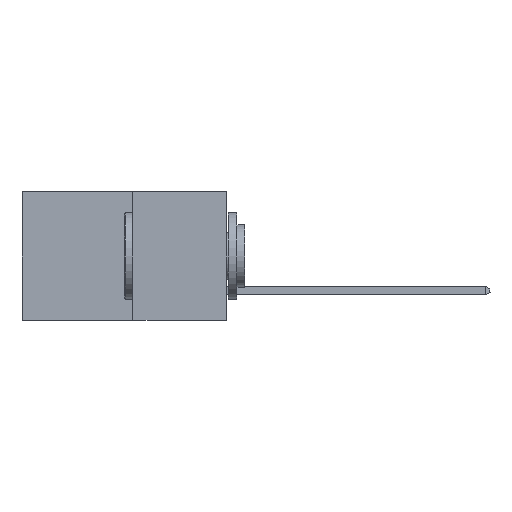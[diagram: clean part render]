
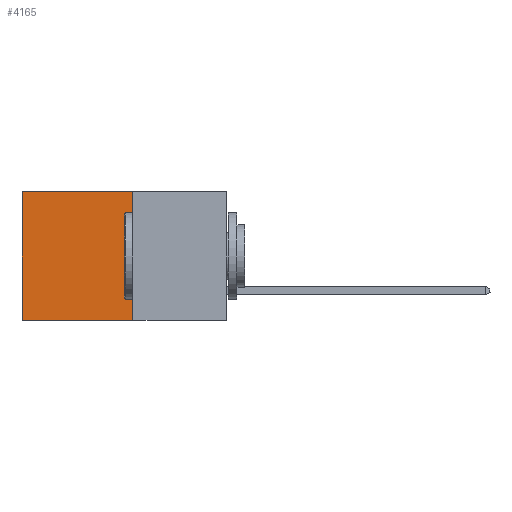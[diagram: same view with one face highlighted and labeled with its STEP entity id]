
A CAD part, left-side view. The second image highlights one B-rep face of the part: STEP entity #4165.
In plain terms, the highlighted planar face has unit normal (-1, 0, 0).
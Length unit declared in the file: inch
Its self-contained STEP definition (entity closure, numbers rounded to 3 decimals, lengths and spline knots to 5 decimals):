
#2106 = ORIENTED_EDGE ( 'NONE', *, *, #10642, .T. ) ;
#2126 = VERTEX_POINT ( 'NONE', #22899 ) ;
#2485 = CARTESIAN_POINT ( 'NONE',  ( 0.277, 0.27, -0.37 ) ) ;
#2646 = DIRECTION ( 'NONE',  ( 0., 0., -1. ) ) ;
#3081 = VECTOR ( 'NONE', #4886, 39.37008 ) ;
#3517 = CARTESIAN_POINT ( 'NONE',  ( 0.277, 0.27, 0. ) ) ;
#4165 = ADVANCED_FACE ( 'NONE', ( #8688 ), #10980, .F. ) ;
#4886 = DIRECTION ( 'NONE',  ( 0., 0., -1. ) ) ;
#5618 = LINE ( 'NONE', #25463, #28935 ) ;
#5661 = ORIENTED_EDGE ( 'NONE', *, *, #24404, .F. ) ;
#6043 = CARTESIAN_POINT ( 'NONE',  ( 0.277, 0.27, -0.37 ) ) ;
#6170 = CARTESIAN_POINT ( 'NONE',  ( 0.277, 0.27, -0.37 ) ) ;
#6928 = CARTESIAN_POINT ( 'NONE',  ( 0.277, 0.59, 0. ) ) ;
#7022 = ORIENTED_EDGE ( 'NONE', *, *, #10318, .T. ) ;
#8307 = LINE ( 'NONE', #17026, #26738 ) ;
#8645 = DIRECTION ( 'NONE',  ( 0., 1., 0. ) ) ;
#8688 = FACE_OUTER_BOUND ( 'NONE', #18865, .T. ) ;
#9369 = VERTEX_POINT ( 'NONE', #6170 ) ;
#10318 = EDGE_CURVE ( 'NONE', #23981, #2126, #8307, .T. ) ;
#10642 = EDGE_CURVE ( 'NONE', #29836, #23981, #5618, .T. ) ;
#10799 = DIRECTION ( 'NONE',  ( 0., 0., -1. ) ) ;
#10828 = DIRECTION ( 'NONE',  ( 1., 0., 0. ) ) ;
#10940 = CARTESIAN_POINT ( 'NONE',  ( 0.277, 0.27, -0.37 ) ) ;
#10980 = PLANE ( 'NONE',  #31040 ) ;
#17026 = CARTESIAN_POINT ( 'NONE',  ( 0.277, 0.59, -0.37 ) ) ;
#18005 = DIRECTION ( 'NONE',  ( 0., 1., 0. ) ) ;
#18865 = EDGE_LOOP ( 'NONE', ( #7022, #5661, #30548, #2106 ) ) ;
#22899 = CARTESIAN_POINT ( 'NONE',  ( 0.277, 0.59, -0.37 ) ) ;
#22957 = VECTOR ( 'NONE', #18005, 39.37008 ) ;
#23981 = VERTEX_POINT ( 'NONE', #6928 ) ;
#24404 = EDGE_CURVE ( 'NONE', #9369, #2126, #28544, .T. ) ;
#25463 = CARTESIAN_POINT ( 'NONE',  ( 0.277, 0.27, 0. ) ) ;
#26738 = VECTOR ( 'NONE', #2646, 39.37008 ) ;
#27566 = LINE ( 'NONE', #2485, #3081 ) ;
#27576 = EDGE_CURVE ( 'NONE', #29836, #9369, #27566, .T. ) ;
#28544 = LINE ( 'NONE', #6043, #22957 ) ;
#28935 = VECTOR ( 'NONE', #8645, 39.37008 ) ;
#29836 = VERTEX_POINT ( 'NONE', #3517 ) ;
#30548 = ORIENTED_EDGE ( 'NONE', *, *, #27576, .F. ) ;
#31040 = AXIS2_PLACEMENT_3D ( 'NONE', #10940, #10828, #10799 ) ;
